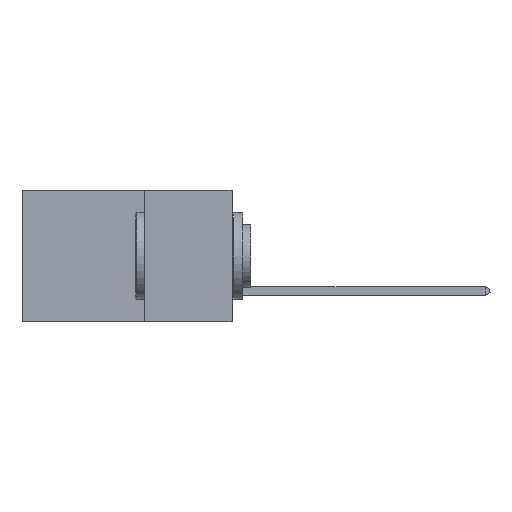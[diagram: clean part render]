
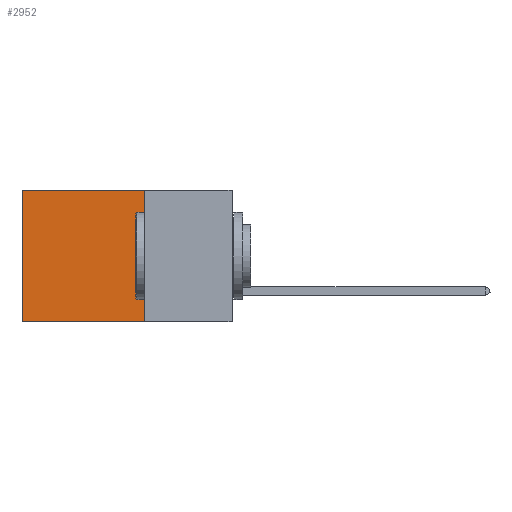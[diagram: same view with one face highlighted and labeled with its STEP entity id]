
A CAD part, left-side view. The second image highlights one B-rep face of the part: STEP entity #2952.
In plain terms, the highlighted planar face has unit normal (-1, 0, 0).
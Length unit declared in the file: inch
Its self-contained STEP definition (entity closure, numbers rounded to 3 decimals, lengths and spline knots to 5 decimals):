
#392 = LINE ( 'NONE', #1490, #6835 ) ;
#612 = DIRECTION ( 'NONE',  ( 0., 1., 0. ) ) ;
#996 = LINE ( 'NONE', #5197, #13215 ) ;
#1490 = CARTESIAN_POINT ( 'NONE',  ( 0.2875, 0.6, -0.375 ) ) ;
#1958 = CARTESIAN_POINT ( 'NONE',  ( 0.2875, 0.25, -0.375 ) ) ;
#1973 = EDGE_CURVE ( 'NONE', #12703, #9478, #392, .T. ) ;
#2288 = EDGE_CURVE ( 'NONE', #3555, #6491, #13609, .T. ) ;
#2289 = DIRECTION ( 'NONE',  ( 0., 0., -1. ) ) ;
#2296 = VECTOR ( 'NONE', #6601, 39.37008 ) ;
#2401 = CARTESIAN_POINT ( 'NONE',  ( 0.2875, 0.6, 0. ) ) ;
#2521 = EDGE_LOOP ( 'NONE', ( #4570, #5752, #2776, #10425 ) ) ;
#2776 = ORIENTED_EDGE ( 'NONE', *, *, #2288, .F. ) ;
#2886 = AXIS2_PLACEMENT_3D ( 'NONE', #8483, #12691, #2289 ) ;
#2952 = ADVANCED_FACE ( 'NONE', ( #11731 ), #9523, .F. ) ;
#2996 = DIRECTION ( 'NONE',  ( 0., 0., -1. ) ) ;
#3555 = VERTEX_POINT ( 'NONE', #10050 ) ;
#3662 = LINE ( 'NONE', #7711, #2296 ) ;
#4570 = ORIENTED_EDGE ( 'NONE', *, *, #1973, .T. ) ;
#5197 = CARTESIAN_POINT ( 'NONE',  ( 0.2875, 0.25, -0.375 ) ) ;
#5752 = ORIENTED_EDGE ( 'NONE', *, *, #9915, .F. ) ;
#6491 = VERTEX_POINT ( 'NONE', #9338 ) ;
#6601 = DIRECTION ( 'NONE',  ( 0., 1., 0. ) ) ;
#6649 = DIRECTION ( 'NONE',  ( 0., 0., -1. ) ) ;
#6835 = VECTOR ( 'NONE', #6649, 39.37008 ) ;
#7711 = CARTESIAN_POINT ( 'NONE',  ( 0.2875, 0.25, 0. ) ) ;
#8483 = CARTESIAN_POINT ( 'NONE',  ( 0.2875, 0.25, -0.375 ) ) ;
#9297 = CARTESIAN_POINT ( 'NONE',  ( 0.2875, 0.6, -0.375 ) ) ;
#9338 = CARTESIAN_POINT ( 'NONE',  ( 0.2875, 0.25, -0.375 ) ) ;
#9478 = VERTEX_POINT ( 'NONE', #9297 ) ;
#9523 = PLANE ( 'NONE',  #2886 ) ;
#9915 = EDGE_CURVE ( 'NONE', #6491, #9478, #996, .T. ) ;
#10050 = CARTESIAN_POINT ( 'NONE',  ( 0.2875, 0.25, 0. ) ) ;
#10425 = ORIENTED_EDGE ( 'NONE', *, *, #12371, .T. ) ;
#10813 = VECTOR ( 'NONE', #2996, 39.37008 ) ;
#11731 = FACE_OUTER_BOUND ( 'NONE', #2521, .T. ) ;
#12371 = EDGE_CURVE ( 'NONE', #3555, #12703, #3662, .T. ) ;
#12691 = DIRECTION ( 'NONE',  ( 1., 0., 0. ) ) ;
#12703 = VERTEX_POINT ( 'NONE', #2401 ) ;
#13215 = VECTOR ( 'NONE', #612, 39.37008 ) ;
#13609 = LINE ( 'NONE', #1958, #10813 ) ;
